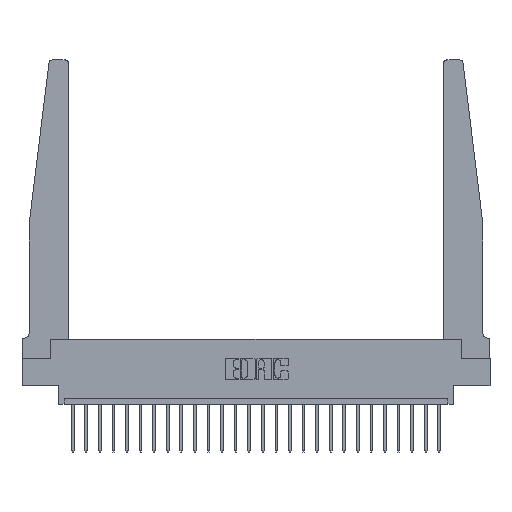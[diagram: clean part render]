
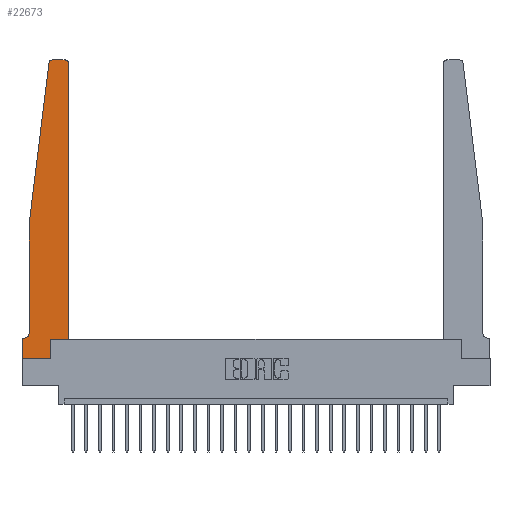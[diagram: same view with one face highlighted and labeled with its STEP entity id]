
A CAD part, top view. The second image highlights one B-rep face of the part: STEP entity #22673.
In plain terms, the highlighted planar face has unit normal (0, 0, 1).
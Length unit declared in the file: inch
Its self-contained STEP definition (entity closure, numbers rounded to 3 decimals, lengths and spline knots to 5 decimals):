
#520 = EDGE_CURVE ( 'NONE', #20060, #17224, #16636, .T. ) ;
#756 = VERTEX_POINT ( 'NONE', #16720 ) ;
#945 = CARTESIAN_POINT ( 'NONE',  ( 0.425, 0.18, 0.37 ) ) ;
#967 = CARTESIAN_POINT ( 'NONE',  ( 0.065, 1.25, 0.37 ) ) ;
#1376 = DIRECTION ( 'NONE',  ( -1., 0., 0. ) ) ;
#1616 = EDGE_CURVE ( 'NONE', #16429, #20060, #17526, .T. ) ;
#1738 = DIRECTION ( 'NONE',  ( 1., 0., 0. ) ) ;
#1805 = ORIENTED_EDGE ( 'NONE', *, *, #1616, .T. ) ;
#1967 = ORIENTED_EDGE ( 'NONE', *, *, #520, .T. ) ;
#2140 = DIRECTION ( 'NONE',  ( -1., 0., 0. ) ) ;
#2412 = EDGE_CURVE ( 'NONE', #9722, #19420, #12175, .T. ) ;
#3072 = CARTESIAN_POINT ( 'NONE',  ( 0.2605, 0., 0.37 ) ) ;
#3103 = CARTESIAN_POINT ( 'NONE',  ( 0.25, 2.75, 0.37 ) ) ;
#3284 = EDGE_CURVE ( 'NONE', #17224, #9144, #13741, .T. ) ;
#3725 = CARTESIAN_POINT ( 'NONE',  ( 0., 0.1875, 0.37 ) ) ;
#3896 = CIRCLE ( 'NONE', #9886, 0.03 ) ;
#4445 = DIRECTION ( 'NONE',  ( 0., 1., 0. ) ) ;
#4569 = VECTOR ( 'NONE', #13901, 39.37008 ) ;
#4757 = DIRECTION ( 'NONE',  ( 1., 0., 0. ) ) ;
#4824 = EDGE_CURVE ( 'NONE', #9144, #9722, #10401, .T. ) ;
#5089 = VERTEX_POINT ( 'NONE', #21095 ) ;
#5155 = CARTESIAN_POINT ( 'NONE',  ( 0., 0., 0.37 ) ) ;
#5992 = CARTESIAN_POINT ( 'NONE',  ( 0.2605, 0.18, 0.37 ) ) ;
#6034 = CARTESIAN_POINT ( 'NONE',  ( 0.065, 1.25, 0.37 ) ) ;
#6059 = CARTESIAN_POINT ( 'NONE',  ( 0.27653, 2.72, 0.37 ) ) ;
#6189 = ORIENTED_EDGE ( 'NONE', *, *, #23565, .T. ) ;
#7607 = CARTESIAN_POINT ( 'NONE',  ( 0.425, 2.72, 0.37 ) ) ;
#7830 = ORIENTED_EDGE ( 'NONE', *, *, #20961, .T. ) ;
#7942 = CARTESIAN_POINT ( 'NONE',  ( 0.425, 0.18, 0.37 ) ) ;
#8136 = DIRECTION ( 'NONE',  ( 0., 1., 0. ) ) ;
#8265 = PLANE ( 'NONE',  #14624 ) ;
#8545 = CARTESIAN_POINT ( 'NONE',  ( 0.2605, 0.18, 0.37 ) ) ;
#8602 = VECTOR ( 'NONE', #24260, 39.37008 ) ;
#9067 = VERTEX_POINT ( 'NONE', #17410 ) ;
#9144 = VERTEX_POINT ( 'NONE', #8545 ) ;
#9667 = CIRCLE ( 'NONE', #13646, 0.03 ) ;
#9722 = VERTEX_POINT ( 'NONE', #12857 ) ;
#9832 = DIRECTION ( 'NONE',  ( 0., 0., 1. ) ) ;
#9886 = AXIS2_PLACEMENT_3D ( 'NONE', #6059, #21310, #1738 ) ;
#10033 = EDGE_CURVE ( 'NONE', #16542, #22119, #23150, .T. ) ;
#10165 = DIRECTION ( 'NONE',  ( 0., 0., -1. ) ) ;
#10255 = VECTOR ( 'NONE', #20901, 39.37008 ) ;
#10272 = FACE_OUTER_BOUND ( 'NONE', #11128, .T. ) ;
#10401 = LINE ( 'NONE', #945, #23589 ) ;
#10792 = AXIS2_PLACEMENT_3D ( 'NONE', #19642, #10165, #17758 ) ;
#10871 = VECTOR ( 'NONE', #4445, 39.37008 ) ;
#11128 = EDGE_LOOP ( 'NONE', ( #21236, #6189, #13809, #7830, #11958, #23590, #1805, #1967, #14688, #23438, #21705, #13534 ) ) ;
#11958 = ORIENTED_EDGE ( 'NONE', *, *, #14533, .T. ) ;
#12175 = LINE ( 'NONE', #7942, #10871 ) ;
#12344 = EDGE_CURVE ( 'NONE', #23379, #16429, #24591, .T. ) ;
#12575 = CARTESIAN_POINT ( 'NONE',  ( 0.015, 0.1875, 0.37 ) ) ;
#12857 = CARTESIAN_POINT ( 'NONE',  ( 0.425, 0.18, 0.37 ) ) ;
#13515 = CARTESIAN_POINT ( 'NONE',  ( 0., 0., 0.37 ) ) ;
#13534 = ORIENTED_EDGE ( 'NONE', *, *, #18164, .T. ) ;
#13646 = AXIS2_PLACEMENT_3D ( 'NONE', #17696, #9832, #19304 ) ;
#13741 = LINE ( 'NONE', #5992, #17195 ) ;
#13809 = ORIENTED_EDGE ( 'NONE', *, *, #10033, .T. ) ;
#13901 = DIRECTION ( 'NONE',  ( 0., -1., 0. ) ) ;
#14533 = EDGE_CURVE ( 'NONE', #5089, #23379, #20749, .T. ) ;
#14624 = AXIS2_PLACEMENT_3D ( 'NONE', #15878, #18240, #19624 ) ;
#14688 = ORIENTED_EDGE ( 'NONE', *, *, #3284, .T. ) ;
#15391 = CARTESIAN_POINT ( 'NONE',  ( 0., 0., 0.37 ) ) ;
#15878 = CARTESIAN_POINT ( 'NONE',  ( 0., 0.1875, 0.37 ) ) ;
#15903 = DIRECTION ( 'NONE',  ( 0., -1., 0. ) ) ;
#16262 = LINE ( 'NONE', #967, #20538 ) ;
#16429 = VERTEX_POINT ( 'NONE', #3725 ) ;
#16542 = VERTEX_POINT ( 'NONE', #18072 ) ;
#16636 = LINE ( 'NONE', #5155, #8602 ) ;
#16643 = VECTOR ( 'NONE', #1376, 39.37008 ) ;
#16720 = CARTESIAN_POINT ( 'NONE',  ( 0.395, 2.75, 0.37 ) ) ;
#17195 = VECTOR ( 'NONE', #8136, 39.37008 ) ;
#17224 = VERTEX_POINT ( 'NONE', #3072 ) ;
#17410 = CARTESIAN_POINT ( 'NONE',  ( 0.27653, 2.75, 0.37 ) ) ;
#17526 = LINE ( 'NONE', #15391, #4569 ) ;
#17696 = CARTESIAN_POINT ( 'NONE',  ( 0.395, 2.72, 0.37 ) ) ;
#17758 = DIRECTION ( 'NONE',  ( -1., 0., 0. ) ) ;
#18072 = CARTESIAN_POINT ( 'NONE',  ( 0.24675, 2.72367, 0.37 ) ) ;
#18164 = EDGE_CURVE ( 'NONE', #19420, #756, #9667, .T. ) ;
#18240 = DIRECTION ( 'NONE',  ( 0., 0., 1. ) ) ;
#18334 = LINE ( 'NONE', #3103, #16643 ) ;
#18928 = CARTESIAN_POINT ( 'NONE',  ( 0.065, 1.25, 0.37 ) ) ;
#19090 = VECTOR ( 'NONE', #2140, 39.37008 ) ;
#19304 = DIRECTION ( 'NONE',  ( 1., 0., 0. ) ) ;
#19420 = VERTEX_POINT ( 'NONE', #7607 ) ;
#19624 = DIRECTION ( 'NONE',  ( 1., 0., 0. ) ) ;
#19642 = CARTESIAN_POINT ( 'NONE',  ( 0.015, 0.2375, 0.37 ) ) ;
#20060 = VERTEX_POINT ( 'NONE', #13515 ) ;
#20538 = VECTOR ( 'NONE', #15903, 39.37008 ) ;
#20749 = CIRCLE ( 'NONE', #10792, 0.05 ) ;
#20901 = DIRECTION ( 'NONE',  ( -0.122, -0.992, 0. ) ) ;
#20961 = EDGE_CURVE ( 'NONE', #22119, #5089, #16262, .T. ) ;
#21095 = CARTESIAN_POINT ( 'NONE',  ( 0.065, 0.2375, 0.37 ) ) ;
#21236 = ORIENTED_EDGE ( 'NONE', *, *, #23392, .T. ) ;
#21310 = DIRECTION ( 'NONE',  ( 0., 0., 1. ) ) ;
#21705 = ORIENTED_EDGE ( 'NONE', *, *, #2412, .T. ) ;
#22119 = VERTEX_POINT ( 'NONE', #18928 ) ;
#22673 = ADVANCED_FACE ( 'NONE', ( #10272 ), #8265, .T. ) ;
#23090 = CARTESIAN_POINT ( 'NONE',  ( 0.065, 0.1875, 0.37 ) ) ;
#23150 = LINE ( 'NONE', #6034, #10255 ) ;
#23379 = VERTEX_POINT ( 'NONE', #12575 ) ;
#23392 = EDGE_CURVE ( 'NONE', #756, #9067, #18334, .T. ) ;
#23438 = ORIENTED_EDGE ( 'NONE', *, *, #4824, .T. ) ;
#23565 = EDGE_CURVE ( 'NONE', #9067, #16542, #3896, .T. ) ;
#23589 = VECTOR ( 'NONE', #4757, 39.37008 ) ;
#23590 = ORIENTED_EDGE ( 'NONE', *, *, #12344, .T. ) ;
#24260 = DIRECTION ( 'NONE',  ( 1., 0., 0. ) ) ;
#24591 = LINE ( 'NONE', #23090, #19090 ) ;
